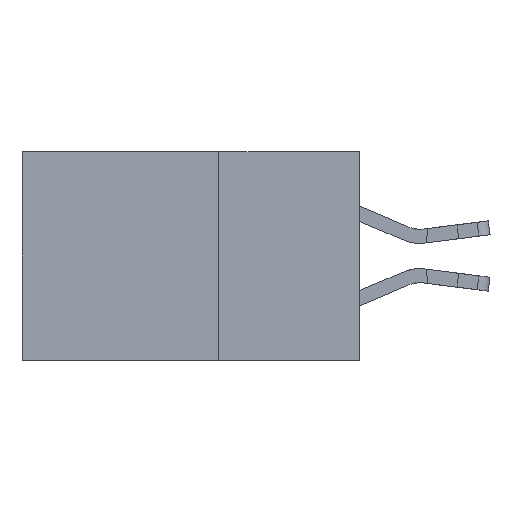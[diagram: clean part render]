
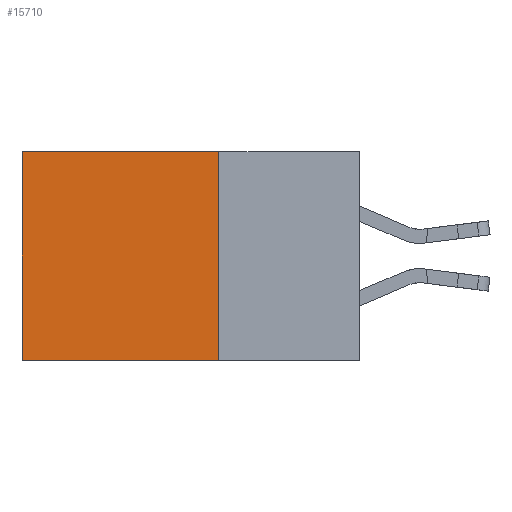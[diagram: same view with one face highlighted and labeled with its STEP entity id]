
A CAD part, left-side view. The second image highlights one B-rep face of the part: STEP entity #15710.
In plain terms, the highlighted planar face has unit normal (-1, 0, 0).
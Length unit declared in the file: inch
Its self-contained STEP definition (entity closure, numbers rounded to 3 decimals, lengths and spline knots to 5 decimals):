
#973 = EDGE_CURVE ( 'NONE', #10685, #1756, #20687, .T. ) ;
#1389 = CARTESIAN_POINT ( 'NONE',  ( 0.2875, 0.6, 0. ) ) ;
#1756 = VERTEX_POINT ( 'NONE', #14334 ) ;
#1789 = VERTEX_POINT ( 'NONE', #11263 ) ;
#2252 = LINE ( 'NONE', #8645, #18594 ) ;
#3300 = EDGE_CURVE ( 'NONE', #1789, #4314, #2252, .T. ) ;
#3467 = ORIENTED_EDGE ( 'NONE', *, *, #17922, .F. ) ;
#4314 = VERTEX_POINT ( 'NONE', #18742 ) ;
#5114 = LINE ( 'NONE', #8151, #5379 ) ;
#5379 = VECTOR ( 'NONE', #9824, 39.37008 ) ;
#5683 = ORIENTED_EDGE ( 'NONE', *, *, #15851, .T. ) ;
#5976 = FACE_OUTER_BOUND ( 'NONE', #18978, .T. ) ;
#6322 = DIRECTION ( 'NONE',  ( 0., 1., 0. ) ) ;
#7438 = VECTOR ( 'NONE', #6322, 39.37008 ) ;
#7772 = DIRECTION ( 'NONE',  ( 0., 0., -1. ) ) ;
#8151 = CARTESIAN_POINT ( 'NONE',  ( 0.2875, 0.25, 0. ) ) ;
#8240 = DIRECTION ( 'NONE',  ( 0., 0., -1. ) ) ;
#8645 = CARTESIAN_POINT ( 'NONE',  ( 0.2875, 0.25, 0. ) ) ;
#9085 = CARTESIAN_POINT ( 'NONE',  ( 0.2875, 0.6, 0. ) ) ;
#9553 = CARTESIAN_POINT ( 'NONE',  ( 0.2875, 0.25, -0.37 ) ) ;
#9824 = DIRECTION ( 'NONE',  ( 0., 1., 0. ) ) ;
#10685 = VERTEX_POINT ( 'NONE', #9085 ) ;
#10976 = DIRECTION ( 'NONE',  ( 0., 0., -1. ) ) ;
#11078 = PLANE ( 'NONE',  #14737 ) ;
#11263 = CARTESIAN_POINT ( 'NONE',  ( 0.2875, 0.25, 0. ) ) ;
#12342 = DIRECTION ( 'NONE',  ( 1., 0., 0. ) ) ;
#14334 = CARTESIAN_POINT ( 'NONE',  ( 0.2875, 0.6, -0.37 ) ) ;
#14737 = AXIS2_PLACEMENT_3D ( 'NONE', #19066, #12342, #10976 ) ;
#15710 = ADVANCED_FACE ( 'NONE', ( #5976 ), #11078, .F. ) ;
#15749 = LINE ( 'NONE', #9553, #7438 ) ;
#15851 = EDGE_CURVE ( 'NONE', #1789, #10685, #5114, .T. ) ;
#17635 = ORIENTED_EDGE ( 'NONE', *, *, #973, .T. ) ;
#17922 = EDGE_CURVE ( 'NONE', #4314, #1756, #15749, .T. ) ;
#18594 = VECTOR ( 'NONE', #8240, 39.37008 ) ;
#18742 = CARTESIAN_POINT ( 'NONE',  ( 0.2875, 0.25, -0.37 ) ) ;
#18978 = EDGE_LOOP ( 'NONE', ( #17635, #3467, #20063, #5683 ) ) ;
#19066 = CARTESIAN_POINT ( 'NONE',  ( 0.2875, 0.25, 0. ) ) ;
#19995 = VECTOR ( 'NONE', #7772, 39.37008 ) ;
#20063 = ORIENTED_EDGE ( 'NONE', *, *, #3300, .F. ) ;
#20687 = LINE ( 'NONE', #1389, #19995 ) ;
